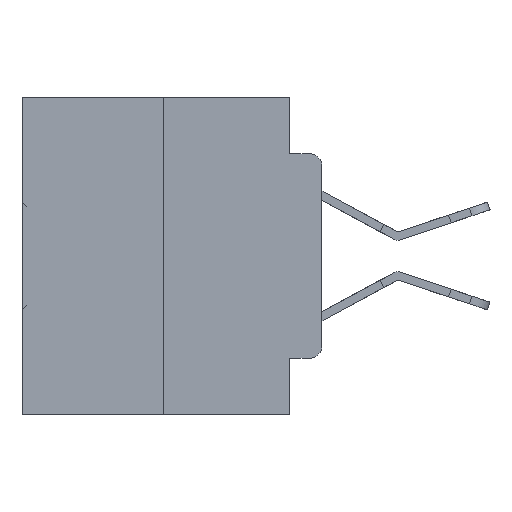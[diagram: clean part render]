
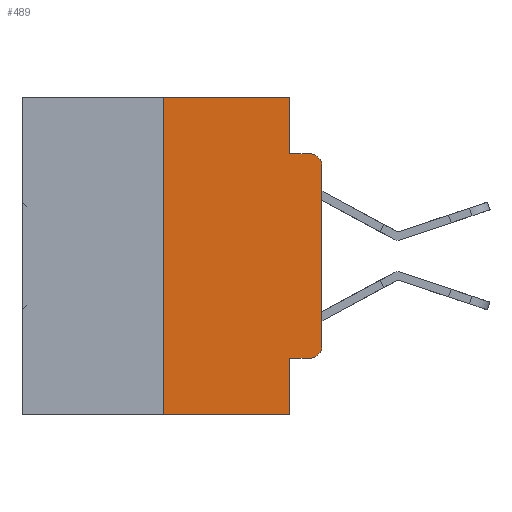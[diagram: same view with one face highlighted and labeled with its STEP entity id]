
A CAD part, left-side view. The second image highlights one B-rep face of the part: STEP entity #489.
In plain terms, the highlighted planar face has unit normal (-1, 0, 0).
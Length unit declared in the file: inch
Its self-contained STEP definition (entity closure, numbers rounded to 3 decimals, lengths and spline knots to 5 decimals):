
#136 = DIRECTION ( 'NONE',  ( -1., 0., 0. ) ) ;
#489 = ADVANCED_FACE ( 'NONE', ( #5194 ), #20323, .F. ) ;
#2378 = EDGE_CURVE ( 'NONE', #15289, #3435, #18007, .T. ) ;
#2493 = EDGE_CURVE ( 'NONE', #3139, #13721, #13777, .T. ) ;
#2640 = CARTESIAN_POINT ( 'NONE',  ( 0., 0.051, -0.4115 ) ) ;
#3129 = CARTESIAN_POINT ( 'NONE',  ( 0., 0., -0.3915 ) ) ;
#3139 = VERTEX_POINT ( 'NONE', #14791 ) ;
#3435 = VERTEX_POINT ( 'NONE', #20347 ) ;
#3695 = EDGE_CURVE ( 'NONE', #20829, #5292, #13267, .T. ) ;
#4394 = EDGE_LOOP ( 'NONE', ( #11451, #35236, #34026, #17010, #15340, #19941, #28882, #15865, #15502, #22953 ) ) ;
#4462 = AXIS2_PLACEMENT_3D ( 'NONE', #12779, #12700, #25142 ) ;
#5194 = FACE_OUTER_BOUND ( 'NONE', #4394, .T. ) ;
#5292 = VERTEX_POINT ( 'NONE', #3129 ) ;
#5674 = CARTESIAN_POINT ( 'NONE',  ( 0., 0.02, -0.1085 ) ) ;
#5716 = DIRECTION ( 'NONE',  ( -1., 0., 0. ) ) ;
#5797 = CARTESIAN_POINT ( 'NONE',  ( 0., 0.051, -0.0885 ) ) ;
#6236 = LINE ( 'NONE', #15366, #26286 ) ;
#6382 = VECTOR ( 'NONE', #30413, 39.37008 ) ;
#6445 = CARTESIAN_POINT ( 'NONE',  ( 0., 0.051, 0. ) ) ;
#6588 = DIRECTION ( 'NONE',  ( 0., 0., -1. ) ) ;
#7753 = VECTOR ( 'NONE', #28813, 39.37008 ) ;
#8184 = EDGE_CURVE ( 'NONE', #33291, #15289, #34474, .T. ) ;
#9111 = DIRECTION ( 'NONE',  ( 0., 0., 1. ) ) ;
#10346 = LINE ( 'NONE', #26347, #23861 ) ;
#11451 = ORIENTED_EDGE ( 'NONE', *, *, #20942, .T. ) ;
#11866 = EDGE_CURVE ( 'NONE', #33291, #27134, #6236, .T. ) ;
#11915 = CARTESIAN_POINT ( 'NONE',  ( 0., 0.25, 0. ) ) ;
#12190 = DIRECTION ( 'NONE',  ( 0., -1., 0. ) ) ;
#12700 = DIRECTION ( 'NONE',  ( 1., 0., 0. ) ) ;
#12779 = CARTESIAN_POINT ( 'NONE',  ( 0., 0.473, 0. ) ) ;
#13267 = CIRCLE ( 'NONE', #21538, 0.02 ) ;
#13271 = CARTESIAN_POINT ( 'NONE',  ( 0., 0.051, -0.4115 ) ) ;
#13586 = LINE ( 'NONE', #13271, #27101 ) ;
#13685 = CARTESIAN_POINT ( 'NONE',  ( 0., 0.473, 0. ) ) ;
#13721 = VERTEX_POINT ( 'NONE', #20606 ) ;
#13777 = CIRCLE ( 'NONE', #20625, 0.02 ) ;
#14791 = CARTESIAN_POINT ( 'NONE',  ( 0., 0., -0.1085 ) ) ;
#14812 = DIRECTION ( 'NONE',  ( 0., 0., -1. ) ) ;
#15082 = CARTESIAN_POINT ( 'NONE',  ( 0., 0.051, -0.5 ) ) ;
#15105 = LINE ( 'NONE', #17911, #7753 ) ;
#15289 = VERTEX_POINT ( 'NONE', #24342 ) ;
#15340 = ORIENTED_EDGE ( 'NONE', *, *, #2378, .F. ) ;
#15366 = CARTESIAN_POINT ( 'NONE',  ( 0., 0.473, -0.5 ) ) ;
#15502 = ORIENTED_EDGE ( 'NONE', *, *, #31205, .T. ) ;
#15865 = ORIENTED_EDGE ( 'NONE', *, *, #23469, .F. ) ;
#16796 = CARTESIAN_POINT ( 'NONE',  ( 0., 0.02, -0.3915 ) ) ;
#17010 = ORIENTED_EDGE ( 'NONE', *, *, #24493, .F. ) ;
#17911 = CARTESIAN_POINT ( 'NONE',  ( 0., 0., 0. ) ) ;
#18007 = LINE ( 'NONE', #13685, #31597 ) ;
#18061 = DIRECTION ( 'NONE',  ( 0., -1., 0. ) ) ;
#18699 = DIRECTION ( 'NONE',  ( 0., -1., 0. ) ) ;
#19438 = CARTESIAN_POINT ( 'NONE',  ( 0., 0.02, -0.4115 ) ) ;
#19512 = DIRECTION ( 'NONE',  ( 0., 0., -1. ) ) ;
#19620 = LINE ( 'NONE', #6445, #33243 ) ;
#19941 = ORIENTED_EDGE ( 'NONE', *, *, #8184, .F. ) ;
#19988 = VECTOR ( 'NONE', #9111, 39.37008 ) ;
#20323 = PLANE ( 'NONE',  #4462 ) ;
#20347 = CARTESIAN_POINT ( 'NONE',  ( 0., 0.051, 0. ) ) ;
#20606 = CARTESIAN_POINT ( 'NONE',  ( 0., 0.02, -0.0885 ) ) ;
#20625 = AXIS2_PLACEMENT_3D ( 'NONE', #5674, #5716, #6588 ) ;
#20829 = VERTEX_POINT ( 'NONE', #19438 ) ;
#20942 = EDGE_CURVE ( 'NONE', #5292, #3139, #15105, .T. ) ;
#21538 = AXIS2_PLACEMENT_3D ( 'NONE', #16796, #136, #19512 ) ;
#21746 = LINE ( 'NONE', #5797, #6382 ) ;
#22953 = ORIENTED_EDGE ( 'NONE', *, *, #3695, .T. ) ;
#23469 = EDGE_CURVE ( 'NONE', #35147, #27134, #10346, .T. ) ;
#23780 = EDGE_CURVE ( 'NONE', #30857, #13721, #21746, .T. ) ;
#23861 = VECTOR ( 'NONE', #31879, 39.37008 ) ;
#24342 = CARTESIAN_POINT ( 'NONE',  ( 0., 0.25, 0. ) ) ;
#24493 = EDGE_CURVE ( 'NONE', #3435, #30857, #19620, .T. ) ;
#25142 = DIRECTION ( 'NONE',  ( 0., 0., -1. ) ) ;
#26286 = VECTOR ( 'NONE', #18061, 39.37008 ) ;
#26347 = CARTESIAN_POINT ( 'NONE',  ( 0., 0.051, 0. ) ) ;
#27101 = VECTOR ( 'NONE', #18699, 39.37008 ) ;
#27134 = VERTEX_POINT ( 'NONE', #15082 ) ;
#27959 = CARTESIAN_POINT ( 'NONE',  ( 0., 0.051, -0.0885 ) ) ;
#28813 = DIRECTION ( 'NONE',  ( 0., 0., 1. ) ) ;
#28882 = ORIENTED_EDGE ( 'NONE', *, *, #11866, .T. ) ;
#30008 = CARTESIAN_POINT ( 'NONE',  ( 0., 0.25, -0.5 ) ) ;
#30413 = DIRECTION ( 'NONE',  ( 0., -1., 0. ) ) ;
#30857 = VERTEX_POINT ( 'NONE', #27959 ) ;
#31205 = EDGE_CURVE ( 'NONE', #35147, #20829, #13586, .T. ) ;
#31597 = VECTOR ( 'NONE', #12190, 39.37008 ) ;
#31879 = DIRECTION ( 'NONE',  ( 0., 0., -1. ) ) ;
#33243 = VECTOR ( 'NONE', #14812, 39.37008 ) ;
#33291 = VERTEX_POINT ( 'NONE', #30008 ) ;
#34026 = ORIENTED_EDGE ( 'NONE', *, *, #23780, .F. ) ;
#34474 = LINE ( 'NONE', #11915, #19988 ) ;
#35147 = VERTEX_POINT ( 'NONE', #2640 ) ;
#35236 = ORIENTED_EDGE ( 'NONE', *, *, #2493, .T. ) ;
